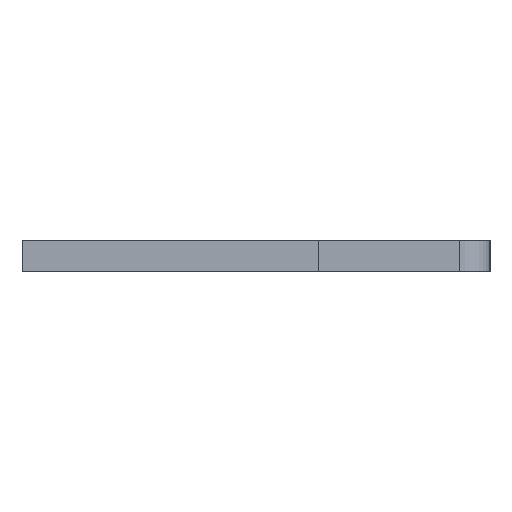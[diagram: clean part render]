
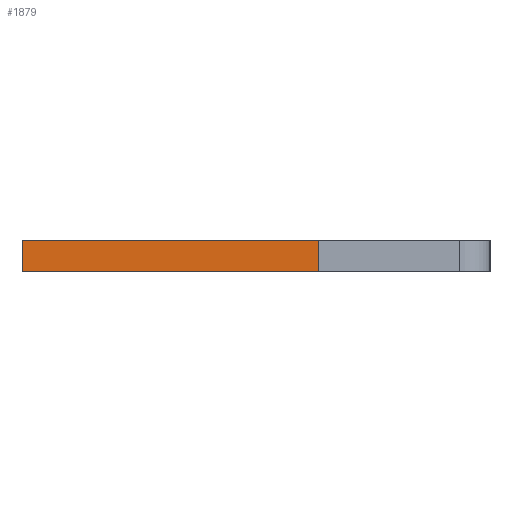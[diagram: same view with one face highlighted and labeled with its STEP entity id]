
A CAD part, left-side view. The second image highlights one B-rep face of the part: STEP entity #1879.
In plain terms, the highlighted face is planar.
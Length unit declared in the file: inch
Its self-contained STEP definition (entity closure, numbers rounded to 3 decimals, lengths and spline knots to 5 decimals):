
#52 = FACE_OUTER_BOUND ( 'NONE', #1948, .T. ) ;
#60 = ORIENTED_EDGE ( 'NONE', *, *, #2752, .T. ) ;
#172 = EDGE_CURVE ( 'NONE', #2248, #2225, #1538, .T. ) ;
#216 = CARTESIAN_POINT ( 'NONE',  ( -0.01, -0.04, -0.04 ) ) ;
#255 = VECTOR ( 'NONE', #2328, 39.37008 ) ;
#386 = VECTOR ( 'NONE', #2429, 39.37008 ) ;
#480 = CARTESIAN_POINT ( 'NONE',  ( 0.01, -0.04, -0.04 ) ) ;
#520 = VERTEX_POINT ( 'NONE', #216 ) ;
#638 = CARTESIAN_POINT ( 'NONE',  ( 0.01, 0.15, -0.04 ) ) ;
#685 = CARTESIAN_POINT ( 'NONE',  ( -0.01, 0.15, -0.04 ) ) ;
#715 = CARTESIAN_POINT ( 'NONE',  ( 0.01, 0.15, -0.04 ) ) ;
#745 = ORIENTED_EDGE ( 'NONE', *, *, #172, .F. ) ;
#842 = EDGE_CURVE ( 'NONE', #520, #1504, #2365, .T. ) ;
#904 = CARTESIAN_POINT ( 'NONE',  ( 0.01, -0.04, -0.04 ) ) ;
#958 = VECTOR ( 'NONE', #1237, 39.37008 ) ;
#1053 = LINE ( 'NONE', #480, #386 ) ;
#1097 = CARTESIAN_POINT ( 'NONE',  ( -0.01, 0.15, -0.04 ) ) ;
#1237 = DIRECTION ( 'NONE',  ( 0., 1., 0. ) ) ;
#1374 = DIRECTION ( 'NONE',  ( 1., 0., 0. ) ) ;
#1504 = VERTEX_POINT ( 'NONE', #1097 ) ;
#1538 = LINE ( 'NONE', #1623, #255 ) ;
#1552 = AXIS2_PLACEMENT_3D ( 'NONE', #2851, #2115, #1374 ) ;
#1623 = CARTESIAN_POINT ( 'NONE',  ( 0.01, 0.15, -0.04 ) ) ;
#1877 = ORIENTED_EDGE ( 'NONE', *, *, #2496, .F. ) ;
#1879 = ADVANCED_FACE ( 'NONE', ( #52 ), #2630, .F. ) ;
#1948 = EDGE_LOOP ( 'NONE', ( #2613, #1877, #745, #60 ) ) ;
#2008 = VECTOR ( 'NONE', #2874, 39.37008 ) ;
#2115 = DIRECTION ( 'NONE',  ( 0., 0., 1. ) ) ;
#2198 = LINE ( 'NONE', #715, #2008 ) ;
#2225 = VERTEX_POINT ( 'NONE', #638 ) ;
#2248 = VERTEX_POINT ( 'NONE', #904 ) ;
#2328 = DIRECTION ( 'NONE',  ( 0., 1., 0. ) ) ;
#2365 = LINE ( 'NONE', #685, #958 ) ;
#2429 = DIRECTION ( 'NONE',  ( -1., 0., 0. ) ) ;
#2496 = EDGE_CURVE ( 'NONE', #2225, #1504, #2198, .T. ) ;
#2613 = ORIENTED_EDGE ( 'NONE', *, *, #842, .T. ) ;
#2630 = PLANE ( 'NONE',  #1552 ) ;
#2752 = EDGE_CURVE ( 'NONE', #2248, #520, #1053, .T. ) ;
#2851 = CARTESIAN_POINT ( 'NONE',  ( 0.01, 0.15, -0.04 ) ) ;
#2874 = DIRECTION ( 'NONE',  ( -1., 0., 0. ) ) ;
